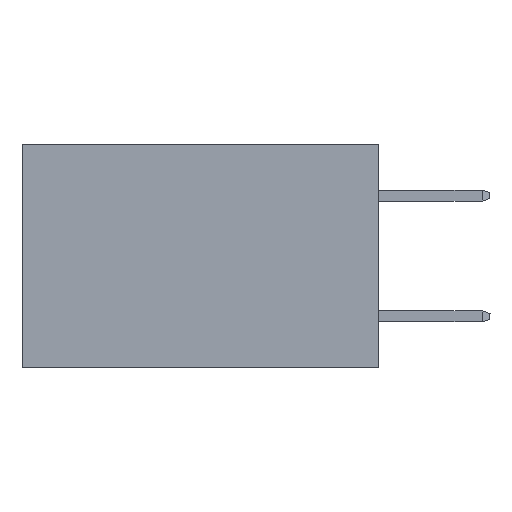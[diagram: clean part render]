
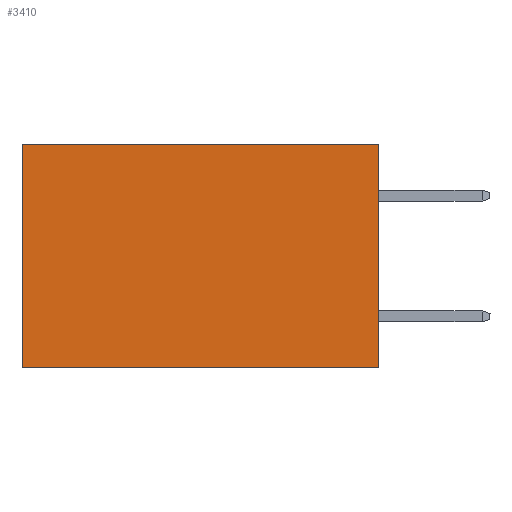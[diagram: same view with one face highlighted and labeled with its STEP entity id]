
A CAD part, left-side view. The second image highlights one B-rep face of the part: STEP entity #3410.
In plain terms, the highlighted planar face has unit normal (-1, 0, 0).
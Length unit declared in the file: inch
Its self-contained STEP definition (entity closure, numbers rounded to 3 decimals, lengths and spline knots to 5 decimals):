
#145 = DIRECTION ( 'NONE',  ( 0., 1., 0. ) ) ;
#584 = VERTEX_POINT ( 'NONE', #5082 ) ;
#678 = VECTOR ( 'NONE', #834, 39.37008 ) ;
#790 = EDGE_CURVE ( 'NONE', #584, #6474, #7458, .T. ) ;
#798 = VECTOR ( 'NONE', #145, 39.37008 ) ;
#814 = EDGE_CURVE ( 'NONE', #9548, #584, #7038, .T. ) ;
#834 = DIRECTION ( 'NONE',  ( 0., 0., -1. ) ) ;
#857 = CARTESIAN_POINT ( 'NONE',  ( 0.277, 0.59, -0.37 ) ) ;
#1155 = CARTESIAN_POINT ( 'NONE',  ( 0.277, 0., -0.37 ) ) ;
#2868 = DIRECTION ( 'NONE',  ( 0., 0., -1. ) ) ;
#2934 = DIRECTION ( 'NONE',  ( 1., 0., 0. ) ) ;
#2963 = CARTESIAN_POINT ( 'NONE',  ( 0.277, 0., -0.37 ) ) ;
#3121 = ORIENTED_EDGE ( 'NONE', *, *, #814, .F. ) ;
#3135 = CARTESIAN_POINT ( 'NONE',  ( 0.277, 0.59, 0. ) ) ;
#3410 = ADVANCED_FACE ( 'NONE', ( #3767 ), #3709, .F. ) ;
#3658 = CARTESIAN_POINT ( 'NONE',  ( 0.277, 0.59, -0.37 ) ) ;
#3709 = PLANE ( 'NONE',  #7868 ) ;
#3718 = CARTESIAN_POINT ( 'NONE',  ( 0.277, 0., 0. ) ) ;
#3767 = FACE_OUTER_BOUND ( 'NONE', #7914, .T. ) ;
#3949 = DIRECTION ( 'NONE',  ( 0., 1., 0. ) ) ;
#4142 = ORIENTED_EDGE ( 'NONE', *, *, #4774, .T. ) ;
#4501 = EDGE_CURVE ( 'NONE', #9548, #5451, #6332, .T. ) ;
#4774 = EDGE_CURVE ( 'NONE', #5451, #6474, #9188, .T. ) ;
#4924 = VECTOR ( 'NONE', #7659, 39.37008 ) ;
#5082 = CARTESIAN_POINT ( 'NONE',  ( 0.277, 0., -0.37 ) ) ;
#5451 = VERTEX_POINT ( 'NONE', #3135 ) ;
#6225 = VECTOR ( 'NONE', #3949, 39.37008 ) ;
#6332 = LINE ( 'NONE', #3718, #6225 ) ;
#6474 = VERTEX_POINT ( 'NONE', #3658 ) ;
#6917 = ORIENTED_EDGE ( 'NONE', *, *, #4501, .T. ) ;
#7038 = LINE ( 'NONE', #8951, #4924 ) ;
#7458 = LINE ( 'NONE', #1155, #798 ) ;
#7659 = DIRECTION ( 'NONE',  ( 0., 0., -1. ) ) ;
#7868 = AXIS2_PLACEMENT_3D ( 'NONE', #2963, #2934, #2868 ) ;
#7914 = EDGE_LOOP ( 'NONE', ( #4142, #9891, #3121, #6917 ) ) ;
#8343 = CARTESIAN_POINT ( 'NONE',  ( 0.277, 0., 0. ) ) ;
#8951 = CARTESIAN_POINT ( 'NONE',  ( 0.277, 0., -0.37 ) ) ;
#9188 = LINE ( 'NONE', #857, #678 ) ;
#9548 = VERTEX_POINT ( 'NONE', #8343 ) ;
#9891 = ORIENTED_EDGE ( 'NONE', *, *, #790, .F. ) ;
